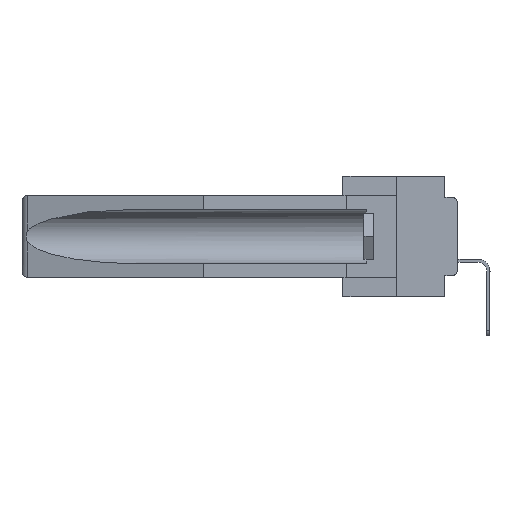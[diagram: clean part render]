
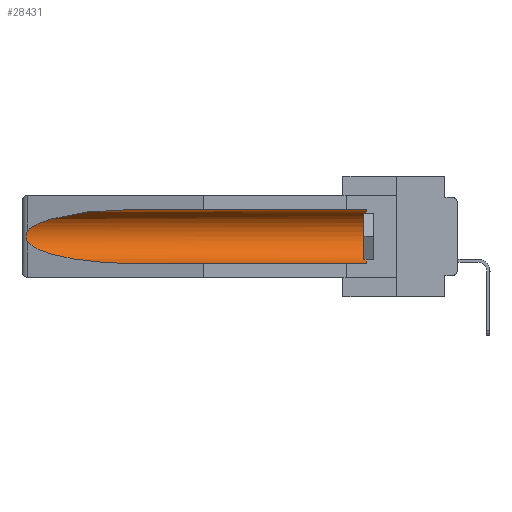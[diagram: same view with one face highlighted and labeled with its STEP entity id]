
A CAD part, left-side view. The second image highlights one B-rep face of the part: STEP entity #28431.
In plain terms, the highlighted cylindrical face has radius 2.857 mm (diameter 5.715 mm), a partial arc.
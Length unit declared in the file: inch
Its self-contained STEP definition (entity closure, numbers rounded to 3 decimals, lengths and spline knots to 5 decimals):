
#60 = EDGE_CURVE ( 'NONE', #1948, #20881, #2413, .T. ) ;
#1608 = EDGE_CURVE ( 'NONE', #20633, #1948, #10630, .T. ) ;
#1948 = VERTEX_POINT ( 'NONE', #21927 ) ;
#2011 = ORIENTED_EDGE ( 'NONE', *, *, #1608, .T. ) ;
#2358 = CARTESIAN_POINT ( 'NONE',  ( 0.26655, 1.53094, -0.18657 ) ) ;
#2413 = B_SPLINE_CURVE_WITH_KNOTS ( 'NONE', 3,
 ( #4700, #13342, #11309, #4506, #2556, #6742, #27014, #2358, #20321, #22685 ),
 .UNSPECIFIED., .F., .F.,
 ( 4, 2, 2, 2, 4 ),
 ( 0., 0.00029, 0.00058, 0.00087, 0.00117 ),
 .UNSPECIFIED. ) ;
#2556 = CARTESIAN_POINT ( 'NONE',  ( 0.2675, 1.53308, -0.16763 ) ) ;
#2784 = CARTESIAN_POINT ( 'NONE',  ( 0.155, 0.126, -0.284 ) ) ;
#2795 = CARTESIAN_POINT ( 'NONE',  ( 0.21114, 1.30732, -0.284 ) ) ;
#3551 = VECTOR ( 'NONE', #3734, 39.37008 ) ;
#3734 = DIRECTION ( 'NONE',  ( 0., 1., 0. ) ) ;
#4506 = CARTESIAN_POINT ( 'NONE',  ( 0.2673, 1.5327, -0.16383 ) ) ;
#4650 = DIRECTION ( 'NONE',  ( 0., 1., 0. ) ) ;
#4700 = CARTESIAN_POINT ( 'NONE',  ( 0.26537, 1.52718, -0.14972 ) ) ;
#5951 = CARTESIAN_POINT ( 'NONE',  ( 0.155, -0.30754, -0.1715 ) ) ;
#6742 = CARTESIAN_POINT ( 'NONE',  ( 0.2675, 1.53308, -0.17534 ) ) ;
#7974 = CARTESIAN_POINT ( 'NONE',  ( 0.155, 0.126, -0.1715 ) ) ;
#8371 = CARTESIAN_POINT ( 'NONE',  ( 0.155, -0.30754, -0.059 ) ) ;
#9506 = CARTESIAN_POINT ( 'NONE',  ( 0.25451, 1.48313, -0.09465 ) ) ;
#9539 = ORIENTED_EDGE ( 'NONE', *, *, #60, .T. ) ;
#10066 = EDGE_CURVE ( 'NONE', #20881, #13789, #14919, .T. ) ;
#10248 = DIRECTION ( 'NONE',  ( 0., 0., 1. ) ) ;
#10572 = CIRCLE ( 'NONE', #24468, 0.1125 ) ;
#10630 =( BOUNDED_CURVE ( )  B_SPLINE_CURVE ( 3, ( #13787, #25298, #9506, #11831 ),
 .UNSPECIFIED., .F., .F. ) 
 B_SPLINE_CURVE_WITH_KNOTS ( ( 4, 4 ),
 ( 4.71239, 6.08839 ),
 .UNSPECIFIED. ) 
 CURVE ( )  GEOMETRIC_REPRESENTATION_ITEM ( )  RATIONAL_B_SPLINE_CURVE ( ( 1., 0.848, 0.848, 1. ) ) 
 REPRESENTATION_ITEM ( '' )  );
#11309 = CARTESIAN_POINT ( 'NONE',  ( 0.26654, 1.53092, -0.15636 ) ) ;
#11616 = EDGE_CURVE ( 'NONE', #19919, #13789, #14068, .T. ) ;
#11721 = CARTESIAN_POINT ( 'NONE',  ( 0.155, 0.126, -0.059 ) ) ;
#11831 = CARTESIAN_POINT ( 'NONE',  ( 0.26537, 1.52718, -0.14972 ) ) ;
#12836 = CARTESIAN_POINT ( 'NONE',  ( 0.155, 1.07973, -0.284 ) ) ;
#12880 = VERTEX_POINT ( 'NONE', #11721 ) ;
#13342 = CARTESIAN_POINT ( 'NONE',  ( 0.26597, 1.52961, -0.15275 ) ) ;
#13787 = CARTESIAN_POINT ( 'NONE',  ( 0.155, 1.07973, -0.059 ) ) ;
#13789 = VERTEX_POINT ( 'NONE', #12836 ) ;
#14068 = LINE ( 'NONE', #22539, #25342 ) ;
#14078 = CARTESIAN_POINT ( 'NONE',  ( 0.155, 1.07973, -0.284 ) ) ;
#14128 = ORIENTED_EDGE ( 'NONE', *, *, #10066, .T. ) ;
#14602 = DIRECTION ( 'NONE',  ( 0., -1., 0. ) ) ;
#14919 =( BOUNDED_CURVE ( )  B_SPLINE_CURVE ( 3, ( #20567, #16124, #2795, #14078 ),
 .UNSPECIFIED., .F., .F. ) 
 B_SPLINE_CURVE_WITH_KNOTS ( ( 4, 4 ),
 ( 0.1948, 1.5708 ),
 .UNSPECIFIED. ) 
 CURVE ( )  GEOMETRIC_REPRESENTATION_ITEM ( )  RATIONAL_B_SPLINE_CURVE ( ( 1., 0.848, 0.848, 1. ) ) 
 REPRESENTATION_ITEM ( '' )  );
#16124 = CARTESIAN_POINT ( 'NONE',  ( 0.25451, 1.48313, -0.24835 ) ) ;
#16566 = ORIENTED_EDGE ( 'NONE', *, *, #16913, .T. ) ;
#16913 = EDGE_CURVE ( 'NONE', #19919, #12880, #10572, .T. ) ;
#18323 = EDGE_CURVE ( 'NONE', #12880, #20633, #22412, .T. ) ;
#19919 = VERTEX_POINT ( 'NONE', #2784 ) ;
#20321 = CARTESIAN_POINT ( 'NONE',  ( 0.26597, 1.5296, -0.19026 ) ) ;
#20567 = CARTESIAN_POINT ( 'NONE',  ( 0.26537, 1.52718, -0.19328 ) ) ;
#20633 = VERTEX_POINT ( 'NONE', #27616 ) ;
#20881 = VERTEX_POINT ( 'NONE', #24052 ) ;
#21687 = CYLINDRICAL_SURFACE ( 'NONE', #25107, 0.1125 ) ;
#21927 = CARTESIAN_POINT ( 'NONE',  ( 0.26537, 1.52718, -0.14972 ) ) ;
#22412 = LINE ( 'NONE', #8371, #3551 ) ;
#22539 = CARTESIAN_POINT ( 'NONE',  ( 0.155, -0.30754, -0.284 ) ) ;
#22685 = CARTESIAN_POINT ( 'NONE',  ( 0.26537, 1.52718, -0.19328 ) ) ;
#23681 = DIRECTION ( 'NONE',  ( 0., 1., 0. ) ) ;
#24052 = CARTESIAN_POINT ( 'NONE',  ( 0.26537, 1.52718, -0.19328 ) ) ;
#24468 = AXIS2_PLACEMENT_3D ( 'NONE', #7974, #14602, #28195 ) ;
#25107 = AXIS2_PLACEMENT_3D ( 'NONE', #5951, #23681, #10248 ) ;
#25298 = CARTESIAN_POINT ( 'NONE',  ( 0.21114, 1.30732, -0.059 ) ) ;
#25342 = VECTOR ( 'NONE', #4650, 39.37008 ) ;
#25927 = FACE_OUTER_BOUND ( 'NONE', #26359, .T. ) ;
#26359 = EDGE_LOOP ( 'NONE', ( #2011, #9539, #14128, #28571, #16566, #26657 ) ) ;
#26657 = ORIENTED_EDGE ( 'NONE', *, *, #18323, .T. ) ;
#27014 = CARTESIAN_POINT ( 'NONE',  ( 0.2673, 1.53269, -0.17917 ) ) ;
#27616 = CARTESIAN_POINT ( 'NONE',  ( 0.155, 1.07973, -0.059 ) ) ;
#28195 = DIRECTION ( 'NONE',  ( 0., 0., 1. ) ) ;
#28431 = ADVANCED_FACE ( 'NONE', ( #25927 ), #21687, .F. ) ;
#28571 = ORIENTED_EDGE ( 'NONE', *, *, #11616, .F. ) ;
